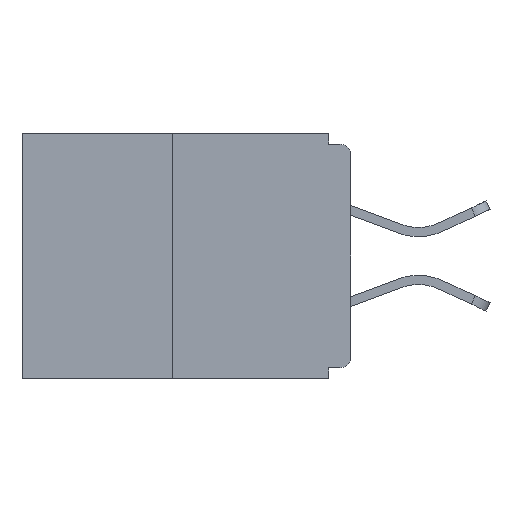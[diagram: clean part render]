
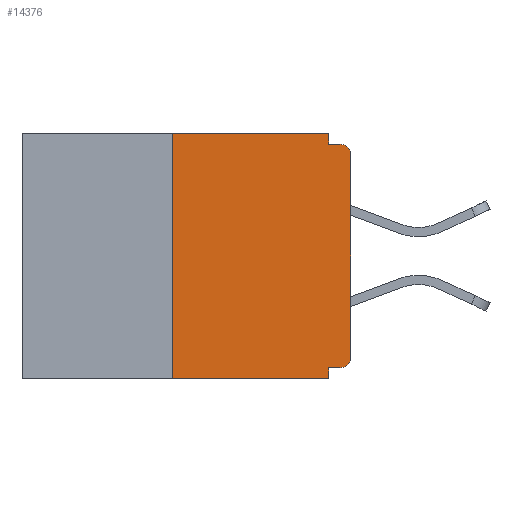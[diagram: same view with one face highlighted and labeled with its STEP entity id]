
A CAD part, left-side view. The second image highlights one B-rep face of the part: STEP entity #14376.
In plain terms, the highlighted planar face has unit normal (-1, 0, 0).
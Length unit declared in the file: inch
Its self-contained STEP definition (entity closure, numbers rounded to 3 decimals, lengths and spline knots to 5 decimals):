
#379 = DIRECTION ( 'NONE',  ( 0., 0., -1. ) ) ;
#629 = VERTEX_POINT ( 'NONE', #5029 ) ;
#966 = DIRECTION ( 'NONE',  ( -1., 0., 0. ) ) ;
#1256 = CARTESIAN_POINT ( 'NONE',  ( 0., 0.031, -0.328 ) ) ;
#1782 = FACE_OUTER_BOUND ( 'NONE', #14328, .T. ) ;
#1902 = LINE ( 'NONE', #6354, #16296 ) ;
#2286 = VERTEX_POINT ( 'NONE', #18907 ) ;
#2441 = CARTESIAN_POINT ( 'NONE',  ( 0., 0., -0.015 ) ) ;
#2448 = LINE ( 'NONE', #2441, #5041 ) ;
#2604 = VERTEX_POINT ( 'NONE', #4302 ) ;
#3964 = CARTESIAN_POINT ( 'NONE',  ( 0., 0., -0.03 ) ) ;
#4166 = CARTESIAN_POINT ( 'NONE',  ( 0., 0.031, 0. ) ) ;
#4302 = CARTESIAN_POINT ( 'NONE',  ( 0., 0.015, -0.328 ) ) ;
#4824 = LINE ( 'NONE', #16800, #20218 ) ;
#5029 = CARTESIAN_POINT ( 'NONE',  ( 0., 0.031, -0.015 ) ) ;
#5041 = VECTOR ( 'NONE', #10608, 39.37008 ) ;
#5565 = VERTEX_POINT ( 'NONE', #12956 ) ;
#5615 = VECTOR ( 'NONE', #379, 39.37008 ) ;
#5683 = AXIS2_PLACEMENT_3D ( 'NONE', #10354, #15330, #13477 ) ;
#5881 = ORIENTED_EDGE ( 'NONE', *, *, #18091, .F. ) ;
#5960 = AXIS2_PLACEMENT_3D ( 'NONE', #10754, #7563, #13033 ) ;
#6086 = EDGE_CURVE ( 'NONE', #9338, #19253, #9660, .T. ) ;
#6161 = CARTESIAN_POINT ( 'NONE',  ( 0., 0.25, -0.343 ) ) ;
#6284 = VECTOR ( 'NONE', #19757, 39.37008 ) ;
#6354 = CARTESIAN_POINT ( 'NONE',  ( 0., 0.031, 0. ) ) ;
#7214 = ORIENTED_EDGE ( 'NONE', *, *, #10140, .F. ) ;
#7563 = DIRECTION ( 'NONE',  ( -1., 0., 0. ) ) ;
#8471 = CARTESIAN_POINT ( 'NONE',  ( 0., 0.25, 0. ) ) ;
#9036 = ORIENTED_EDGE ( 'NONE', *, *, #11698, .F. ) ;
#9140 = VERTEX_POINT ( 'NONE', #4166 ) ;
#9157 = VERTEX_POINT ( 'NONE', #3964 ) ;
#9170 = LINE ( 'NONE', #15510, #20813 ) ;
#9338 = VERTEX_POINT ( 'NONE', #6161 ) ;
#9660 = LINE ( 'NONE', #11909, #14461 ) ;
#9688 = ORIENTED_EDGE ( 'NONE', *, *, #18278, .F. ) ;
#10130 = LINE ( 'NONE', #16597, #5615 ) ;
#10140 = EDGE_CURVE ( 'NONE', #629, #10970, #2448, .T. ) ;
#10354 = CARTESIAN_POINT ( 'NONE',  ( 0., 0.46, 0. ) ) ;
#10565 = LINE ( 'NONE', #8471, #6284 ) ;
#10608 = DIRECTION ( 'NONE',  ( 0., -1., 0. ) ) ;
#10754 = CARTESIAN_POINT ( 'NONE',  ( 0., 0.015, -0.03 ) ) ;
#10821 = CARTESIAN_POINT ( 'NONE',  ( 0., 0.031, -0.343 ) ) ;
#10970 = VERTEX_POINT ( 'NONE', #15588 ) ;
#10991 = VERTEX_POINT ( 'NONE', #1256 ) ;
#11427 = AXIS2_PLACEMENT_3D ( 'NONE', #18545, #966, #18621 ) ;
#11698 = EDGE_CURVE ( 'NONE', #9140, #629, #1902, .T. ) ;
#11724 = ORIENTED_EDGE ( 'NONE', *, *, #17293, .T. ) ;
#11909 = CARTESIAN_POINT ( 'NONE',  ( 0., 0.46, -0.343 ) ) ;
#12423 = CARTESIAN_POINT ( 'NONE',  ( 0., 0.46, 0. ) ) ;
#12480 = CIRCLE ( 'NONE', #11427, 0.015 ) ;
#12700 = ORIENTED_EDGE ( 'NONE', *, *, #15252, .T. ) ;
#12956 = CARTESIAN_POINT ( 'NONE',  ( 0., 0.25, 0. ) ) ;
#13033 = DIRECTION ( 'NONE',  ( 0., 0., -1. ) ) ;
#13201 = LINE ( 'NONE', #12423, #14425 ) ;
#13209 = ORIENTED_EDGE ( 'NONE', *, *, #14324, .F. ) ;
#13477 = DIRECTION ( 'NONE',  ( 0., 0., -1. ) ) ;
#14115 = DIRECTION ( 'NONE',  ( 0., 0., 1. ) ) ;
#14324 = EDGE_CURVE ( 'NONE', #10991, #19253, #10130, .T. ) ;
#14328 = EDGE_LOOP ( 'NONE', ( #5881, #15022, #18500, #13209, #9688, #11724, #20345, #12700, #7214, #9036 ) ) ;
#14376 = ADVANCED_FACE ( 'NONE', ( #1782 ), #18288, .F. ) ;
#14425 = VECTOR ( 'NONE', #20140, 39.37008 ) ;
#14461 = VECTOR ( 'NONE', #19943, 39.37008 ) ;
#15022 = ORIENTED_EDGE ( 'NONE', *, *, #19469, .F. ) ;
#15252 = EDGE_CURVE ( 'NONE', #9157, #10970, #17500, .T. ) ;
#15330 = DIRECTION ( 'NONE',  ( 1., 0., 0. ) ) ;
#15510 = CARTESIAN_POINT ( 'NONE',  ( 0., 0., 0. ) ) ;
#15588 = CARTESIAN_POINT ( 'NONE',  ( 0., 0.015, -0.015 ) ) ;
#16296 = VECTOR ( 'NONE', #17593, 39.37008 ) ;
#16597 = CARTESIAN_POINT ( 'NONE',  ( 0., 0.031, -0.343 ) ) ;
#16725 = EDGE_CURVE ( 'NONE', #2286, #9157, #9170, .T. ) ;
#16800 = CARTESIAN_POINT ( 'NONE',  ( 0., 0., -0.328 ) ) ;
#17293 = EDGE_CURVE ( 'NONE', #2604, #2286, #12480, .T. ) ;
#17500 = CIRCLE ( 'NONE', #5960, 0.015 ) ;
#17593 = DIRECTION ( 'NONE',  ( 0., 0., -1. ) ) ;
#18091 = EDGE_CURVE ( 'NONE', #5565, #9140, #13201, .T. ) ;
#18278 = EDGE_CURVE ( 'NONE', #2604, #10991, #4824, .T. ) ;
#18288 = PLANE ( 'NONE',  #5683 ) ;
#18500 = ORIENTED_EDGE ( 'NONE', *, *, #6086, .T. ) ;
#18545 = CARTESIAN_POINT ( 'NONE',  ( 0., 0.015, -0.313 ) ) ;
#18621 = DIRECTION ( 'NONE',  ( 0., 0., -1. ) ) ;
#18907 = CARTESIAN_POINT ( 'NONE',  ( 0., 0., -0.313 ) ) ;
#19253 = VERTEX_POINT ( 'NONE', #10821 ) ;
#19469 = EDGE_CURVE ( 'NONE', #9338, #5565, #10565, .T. ) ;
#19757 = DIRECTION ( 'NONE',  ( 0., 0., 1. ) ) ;
#19943 = DIRECTION ( 'NONE',  ( 0., -1., 0. ) ) ;
#20140 = DIRECTION ( 'NONE',  ( 0., -1., 0. ) ) ;
#20218 = VECTOR ( 'NONE', #20283, 39.37008 ) ;
#20283 = DIRECTION ( 'NONE',  ( 0., 1., 0. ) ) ;
#20345 = ORIENTED_EDGE ( 'NONE', *, *, #16725, .T. ) ;
#20813 = VECTOR ( 'NONE', #14115, 39.37008 ) ;
